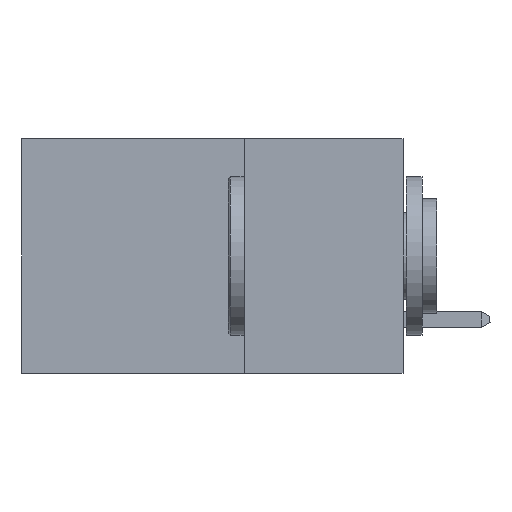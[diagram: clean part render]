
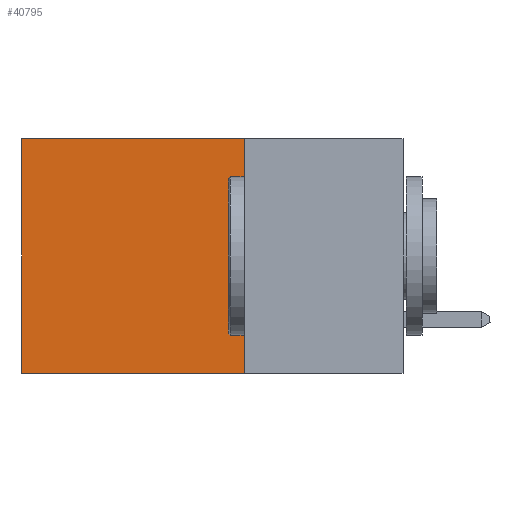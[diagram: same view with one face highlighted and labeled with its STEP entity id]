
A CAD part, left-side view. The second image highlights one B-rep face of the part: STEP entity #40795.
In plain terms, the highlighted planar face has unit normal (-1, 0, 0).
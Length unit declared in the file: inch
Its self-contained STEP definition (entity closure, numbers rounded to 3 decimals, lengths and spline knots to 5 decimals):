
#1103 = LINE ( 'NONE', #21832, #39719 ) ;
#2173 = VECTOR ( 'NONE', #17597, 39.37008 ) ;
#2426 = VERTEX_POINT ( 'NONE', #5107 ) ;
#5107 = CARTESIAN_POINT ( 'NONE',  ( 0.2875, 0.25, -0.37 ) ) ;
#6474 = EDGE_LOOP ( 'NONE', ( #37326, #29456, #40784, #12994 ) ) ;
#8401 = VECTOR ( 'NONE', #27540, 39.37008 ) ;
#8967 = DIRECTION ( 'NONE',  ( 0., 1., 0. ) ) ;
#12859 = EDGE_CURVE ( 'NONE', #16338, #2426, #30339, .T. ) ;
#12994 = ORIENTED_EDGE ( 'NONE', *, *, #13446, .T. ) ;
#13004 = DIRECTION ( 'NONE',  ( 1., 0., 0. ) ) ;
#13202 = VERTEX_POINT ( 'NONE', #27051 ) ;
#13446 = EDGE_CURVE ( 'NONE', #16338, #13202, #1103, .T. ) ;
#15059 = CARTESIAN_POINT ( 'NONE',  ( 0.2875, 0.25, 0. ) ) ;
#16038 = CARTESIAN_POINT ( 'NONE',  ( 0.2875, 0.6, -0.37 ) ) ;
#16338 = VERTEX_POINT ( 'NONE', #31185 ) ;
#16462 = DIRECTION ( 'NONE',  ( 0., 0., -1. ) ) ;
#16817 = EDGE_CURVE ( 'NONE', #13202, #38581, #34955, .T. ) ;
#17597 = DIRECTION ( 'NONE',  ( 0., 1., 0. ) ) ;
#17700 = FACE_OUTER_BOUND ( 'NONE', #6474, .T. ) ;
#18330 = VECTOR ( 'NONE', #34503, 39.37008 ) ;
#19555 = PLANE ( 'NONE',  #39446 ) ;
#21832 = CARTESIAN_POINT ( 'NONE',  ( 0.2875, 0.25, 0. ) ) ;
#25712 = CARTESIAN_POINT ( 'NONE',  ( 0.2875, 0.25, 0. ) ) ;
#27051 = CARTESIAN_POINT ( 'NONE',  ( 0.2875, 0.6, 0. ) ) ;
#27540 = DIRECTION ( 'NONE',  ( 0., 0., -1. ) ) ;
#28199 = EDGE_CURVE ( 'NONE', #2426, #38581, #33779, .T. ) ;
#29456 = ORIENTED_EDGE ( 'NONE', *, *, #28199, .F. ) ;
#30339 = LINE ( 'NONE', #15059, #18330 ) ;
#30878 = CARTESIAN_POINT ( 'NONE',  ( 0.2875, 0.25, -0.37 ) ) ;
#31185 = CARTESIAN_POINT ( 'NONE',  ( 0.2875, 0.25, 0. ) ) ;
#33779 = LINE ( 'NONE', #30878, #2173 ) ;
#34503 = DIRECTION ( 'NONE',  ( 0., 0., -1. ) ) ;
#34955 = LINE ( 'NONE', #39753, #8401 ) ;
#37326 = ORIENTED_EDGE ( 'NONE', *, *, #16817, .T. ) ;
#38581 = VERTEX_POINT ( 'NONE', #16038 ) ;
#39446 = AXIS2_PLACEMENT_3D ( 'NONE', #25712, #13004, #16462 ) ;
#39719 = VECTOR ( 'NONE', #8967, 39.37008 ) ;
#39753 = CARTESIAN_POINT ( 'NONE',  ( 0.2875, 0.6, 0. ) ) ;
#40784 = ORIENTED_EDGE ( 'NONE', *, *, #12859, .F. ) ;
#40795 = ADVANCED_FACE ( 'NONE', ( #17700 ), #19555, .F. ) ;
